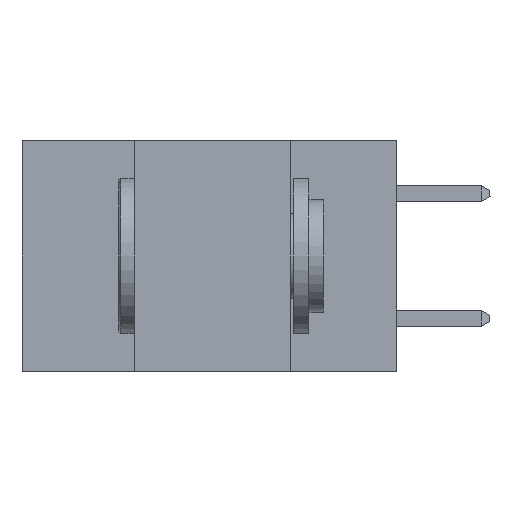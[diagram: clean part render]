
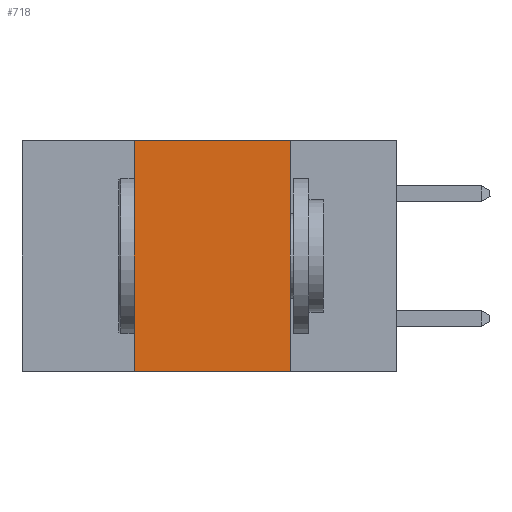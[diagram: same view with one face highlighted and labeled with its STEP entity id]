
A CAD part, left-side view. The second image highlights one B-rep face of the part: STEP entity #718.
In plain terms, the highlighted planar face has unit normal (-1, 0, 0).
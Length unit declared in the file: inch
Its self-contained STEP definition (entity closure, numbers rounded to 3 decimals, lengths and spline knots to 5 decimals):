
#259 = EDGE_CURVE ( 'NONE', #28021, #25524, #5460, .T. ) ;
#718 = ADVANCED_FACE ( 'NONE', ( #6159 ), #22230, .F. ) ;
#1392 = VECTOR ( 'NONE', #25632, 39.37008 ) ;
#1940 = DIRECTION ( 'NONE',  ( 0., 0., 1. ) ) ;
#2383 = VECTOR ( 'NONE', #1940, 39.37008 ) ;
#2520 = CARTESIAN_POINT ( 'NONE',  ( 0., 0.17, 0. ) ) ;
#3129 = CARTESIAN_POINT ( 'NONE',  ( 0., 0.42, 0. ) ) ;
#3391 = DIRECTION ( 'NONE',  ( 1., 0., 0. ) ) ;
#4097 = CARTESIAN_POINT ( 'NONE',  ( 0., 0.17, -0.37 ) ) ;
#4869 = LINE ( 'NONE', #6773, #22742 ) ;
#5460 = LINE ( 'NONE', #28012, #9120 ) ;
#6159 = FACE_OUTER_BOUND ( 'NONE', #24326, .T. ) ;
#6715 = ORIENTED_EDGE ( 'NONE', *, *, #10343, .F. ) ;
#6773 = CARTESIAN_POINT ( 'NONE',  ( 0., 0.6, 0. ) ) ;
#9120 = VECTOR ( 'NONE', #13808, 39.37008 ) ;
#9425 = CARTESIAN_POINT ( 'NONE',  ( 0., 0.6, -0.37 ) ) ;
#10343 = EDGE_CURVE ( 'NONE', #27985, #13997, #22786, .T. ) ;
#11517 = ORIENTED_EDGE ( 'NONE', *, *, #259, .F. ) ;
#13534 = AXIS2_PLACEMENT_3D ( 'NONE', #17285, #3391, #24573 ) ;
#13808 = DIRECTION ( 'NONE',  ( 0., 0., -1. ) ) ;
#13847 = EDGE_CURVE ( 'NONE', #27985, #25524, #15204, .T. ) ;
#13997 = VERTEX_POINT ( 'NONE', #3129 ) ;
#15204 = LINE ( 'NONE', #9425, #1392 ) ;
#15836 = CARTESIAN_POINT ( 'NONE',  ( 0., 0.42, 0. ) ) ;
#17285 = CARTESIAN_POINT ( 'NONE',  ( 0., 0.6, 0. ) ) ;
#20919 = ORIENTED_EDGE ( 'NONE', *, *, #27083, .F. ) ;
#22230 = PLANE ( 'NONE',  #13534 ) ;
#22605 = ORIENTED_EDGE ( 'NONE', *, *, #13847, .T. ) ;
#22742 = VECTOR ( 'NONE', #29811, 39.37008 ) ;
#22786 = LINE ( 'NONE', #15836, #2383 ) ;
#24326 = EDGE_LOOP ( 'NONE', ( #11517, #20919, #6715, #22605 ) ) ;
#24573 = DIRECTION ( 'NONE',  ( 0., 0., -1. ) ) ;
#25524 = VERTEX_POINT ( 'NONE', #4097 ) ;
#25632 = DIRECTION ( 'NONE',  ( 0., -1., 0. ) ) ;
#27083 = EDGE_CURVE ( 'NONE', #13997, #28021, #4869, .T. ) ;
#27985 = VERTEX_POINT ( 'NONE', #30037 ) ;
#28012 = CARTESIAN_POINT ( 'NONE',  ( 0., 0.17, 0. ) ) ;
#28021 = VERTEX_POINT ( 'NONE', #2520 ) ;
#29811 = DIRECTION ( 'NONE',  ( 0., -1., 0. ) ) ;
#30037 = CARTESIAN_POINT ( 'NONE',  ( 0., 0.42, -0.37 ) ) ;
